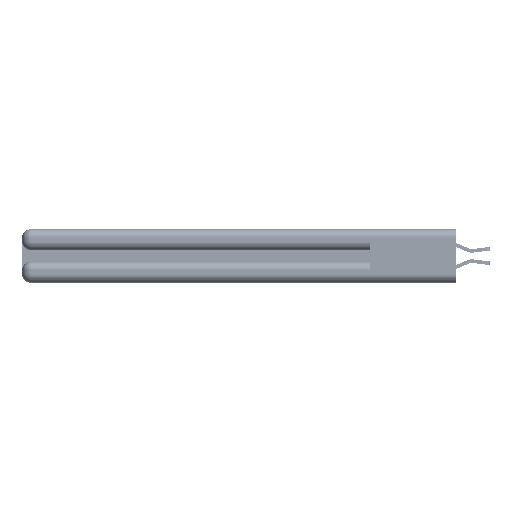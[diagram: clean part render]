
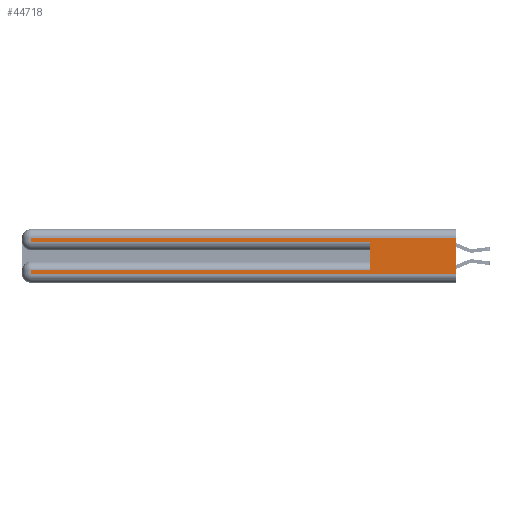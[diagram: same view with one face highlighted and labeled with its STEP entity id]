
A CAD part, left-side view. The second image highlights one B-rep face of the part: STEP entity #44718.
In plain terms, the highlighted planar face has unit normal (-1, 0, 0).
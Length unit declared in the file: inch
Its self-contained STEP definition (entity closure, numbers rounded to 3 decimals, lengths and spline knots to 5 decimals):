
#1966 = VERTEX_POINT ( 'NONE', #45706 ) ;
#2088 = CARTESIAN_POINT ( 'NONE',  ( 0., 2.94, 0.37 ) ) ;
#2801 = CARTESIAN_POINT ( 'NONE',  ( 0., 2.94, 0.37 ) ) ;
#2906 = CARTESIAN_POINT ( 'NONE',  ( 0., 2.94, 0.06 ) ) ;
#3089 = ORIENTED_EDGE ( 'NONE', *, *, #13454, .F. ) ;
#3256 = CARTESIAN_POINT ( 'NONE',  ( 0., 0.6, 0.285 ) ) ;
#4471 = ORIENTED_EDGE ( 'NONE', *, *, #20337, .T. ) ;
#5392 = LINE ( 'NONE', #2088, #45367 ) ;
#5626 = CARTESIAN_POINT ( 'NONE',  ( 0., 0., 0.085 ) ) ;
#7629 = VECTOR ( 'NONE', #17883, 39.37008 ) ;
#8070 = VERTEX_POINT ( 'NONE', #32731 ) ;
#8505 = DIRECTION ( 'NONE',  ( 0., 0., -1. ) ) ;
#8735 = LINE ( 'NONE', #42176, #44544 ) ;
#9004 = VECTOR ( 'NONE', #24574, 39.37008 ) ;
#10439 = LINE ( 'NONE', #2801, #24775 ) ;
#11119 = EDGE_CURVE ( 'NONE', #32857, #28463, #48350, .T. ) ;
#12227 = EDGE_CURVE ( 'NONE', #12501, #28463, #25768, .T. ) ;
#12501 = VERTEX_POINT ( 'NONE', #19379 ) ;
#13137 = VERTEX_POINT ( 'NONE', #2906 ) ;
#13256 = EDGE_LOOP ( 'NONE', ( #3089, #35772, #49615, #19329, #20623, #4471, #16333, #45480 ) ) ;
#13454 = EDGE_CURVE ( 'NONE', #33204, #1966, #31138, .T. ) ;
#13498 = CARTESIAN_POINT ( 'NONE',  ( 0., 0.6, 0.145 ) ) ;
#13515 = VERTEX_POINT ( 'NONE', #28894 ) ;
#16217 = LINE ( 'NONE', #5626, #19277 ) ;
#16333 = ORIENTED_EDGE ( 'NONE', *, *, #19985, .T. ) ;
#17131 = CARTESIAN_POINT ( 'NONE',  ( 0., 0., 0.31 ) ) ;
#17524 = CARTESIAN_POINT ( 'NONE',  ( 0., 0., 0.31 ) ) ;
#17883 = DIRECTION ( 'NONE',  ( 0., 0., 1. ) ) ;
#19169 = VECTOR ( 'NONE', #30049, 39.37008 ) ;
#19277 = VECTOR ( 'NONE', #43753, 39.37008 ) ;
#19282 = LINE ( 'NONE', #17131, #9004 ) ;
#19329 = ORIENTED_EDGE ( 'NONE', *, *, #11119, .T. ) ;
#19379 = CARTESIAN_POINT ( 'NONE',  ( 0., 0.6, 0.085 ) ) ;
#19985 = EDGE_CURVE ( 'NONE', #13515, #13137, #10439, .T. ) ;
#20337 = EDGE_CURVE ( 'NONE', #12501, #13515, #16217, .T. ) ;
#20537 = EDGE_CURVE ( 'NONE', #8070, #32857, #5392, .T. ) ;
#20623 = ORIENTED_EDGE ( 'NONE', *, *, #12227, .F. ) ;
#21790 = DIRECTION ( 'NONE',  ( 0., 0., -1. ) ) ;
#21847 = DIRECTION ( 'NONE',  ( 0., 0., -1. ) ) ;
#22784 = CARTESIAN_POINT ( 'NONE',  ( 0., 2.94, 0.285 ) ) ;
#23879 = DIRECTION ( 'NONE',  ( 1., 0., 0. ) ) ;
#24374 = CARTESIAN_POINT ( 'NONE',  ( 0., 0., 0.37 ) ) ;
#24574 = DIRECTION ( 'NONE',  ( 0., 1., 0. ) ) ;
#24775 = VECTOR ( 'NONE', #21847, 39.37008 ) ;
#25768 = LINE ( 'NONE', #13498, #7629 ) ;
#28463 = VERTEX_POINT ( 'NONE', #3256 ) ;
#28894 = CARTESIAN_POINT ( 'NONE',  ( 0., 2.94, 0.085 ) ) ;
#30049 = DIRECTION ( 'NONE',  ( 0., -1., 0. ) ) ;
#31138 = LINE ( 'NONE', #35706, #45108 ) ;
#32731 = CARTESIAN_POINT ( 'NONE',  ( 0., 2.94, 0.31 ) ) ;
#32857 = VERTEX_POINT ( 'NONE', #22784 ) ;
#33204 = VERTEX_POINT ( 'NONE', #17524 ) ;
#35706 = CARTESIAN_POINT ( 'NONE',  ( 0., 0., 0.37 ) ) ;
#35772 = ORIENTED_EDGE ( 'NONE', *, *, #37364, .T. ) ;
#37364 = EDGE_CURVE ( 'NONE', #33204, #8070, #19282, .T. ) ;
#37953 = EDGE_CURVE ( 'NONE', #13137, #1966, #8735, .T. ) ;
#38199 = CARTESIAN_POINT ( 'NONE',  ( 0., 0., 0.285 ) ) ;
#39260 = DIRECTION ( 'NONE',  ( 0., 0., -1. ) ) ;
#40180 = PLANE ( 'NONE',  #42057 ) ;
#42009 = DIRECTION ( 'NONE',  ( 0., -1., 0. ) ) ;
#42057 = AXIS2_PLACEMENT_3D ( 'NONE', #24374, #23879, #8505 ) ;
#42176 = CARTESIAN_POINT ( 'NONE',  ( 0., 0., 0.06 ) ) ;
#43753 = DIRECTION ( 'NONE',  ( 0., 1., 0. ) ) ;
#44544 = VECTOR ( 'NONE', #42009, 39.37008 ) ;
#44718 = ADVANCED_FACE ( 'NONE', ( #47247 ), #40180, .F. ) ;
#45108 = VECTOR ( 'NONE', #39260, 39.37008 ) ;
#45367 = VECTOR ( 'NONE', #21790, 39.37008 ) ;
#45480 = ORIENTED_EDGE ( 'NONE', *, *, #37953, .T. ) ;
#45706 = CARTESIAN_POINT ( 'NONE',  ( 0., 0., 0.06 ) ) ;
#47247 = FACE_OUTER_BOUND ( 'NONE', #13256, .T. ) ;
#48350 = LINE ( 'NONE', #38199, #19169 ) ;
#49615 = ORIENTED_EDGE ( 'NONE', *, *, #20537, .T. ) ;
